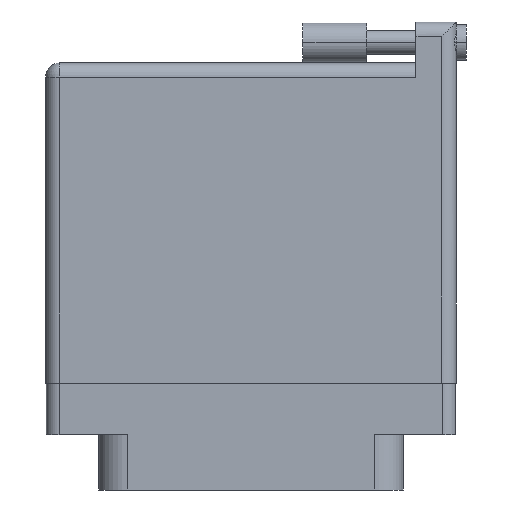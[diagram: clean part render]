
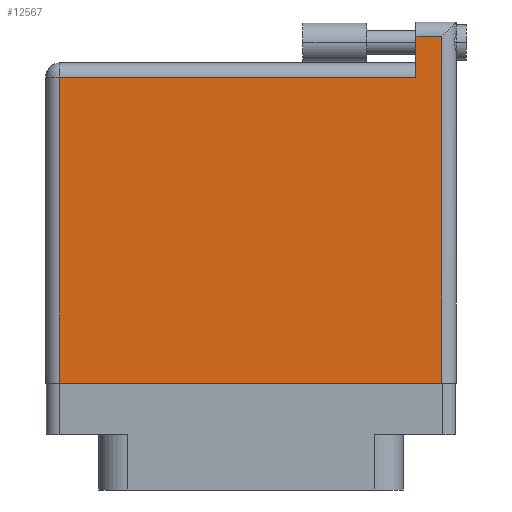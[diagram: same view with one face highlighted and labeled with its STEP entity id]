
A CAD part, front view. The second image highlights one B-rep face of the part: STEP entity #12567.
In plain terms, the highlighted face is planar.
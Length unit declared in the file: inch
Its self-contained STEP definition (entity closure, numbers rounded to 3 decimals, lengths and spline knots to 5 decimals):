
#1122 = AXIS2_PLACEMENT_3D ( 'NONE', #3844, #20524, #31777 ) ;
#2271 = CARTESIAN_POINT ( 'NONE',  ( -1.004, -0.1, 0.4495 ) ) ;
#3331 = CARTESIAN_POINT ( 'NONE',  ( 0.807, 1.396, 0.4495 ) ) ;
#3644 = VERTEX_POINT ( 'NONE', #14735 ) ;
#3844 = CARTESIAN_POINT ( 'NONE',  ( -1.004, 1.466, 0.4495 ) ) ;
#4239 = LINE ( 'NONE', #25022, #27142 ) ;
#4873 = CARTESIAN_POINT ( 'NONE',  ( -0.934, 1.396, 0.4495 ) ) ;
#5853 = EDGE_CURVE ( 'NONE', #35288, #7859, #4239, .T. ) ;
#6407 = LINE ( 'NONE', #24584, #34518 ) ;
#7729 = VECTOR ( 'NONE', #14345, 39.37008 ) ;
#7859 = VERTEX_POINT ( 'NONE', #13746 ) ;
#8720 = CARTESIAN_POINT ( 'NONE',  ( -1.004, 1.596, 0.4495 ) ) ;
#10800 = DIRECTION ( 'NONE',  ( -1., 0., 0. ) ) ;
#11181 = LINE ( 'NONE', #2271, #7729 ) ;
#11555 = EDGE_CURVE ( 'NONE', #15676, #23995, #20229, .T. ) ;
#11770 = DIRECTION ( 'NONE',  ( 0., -1., 0. ) ) ;
#12567 = ADVANCED_FACE ( 'NONE', ( #20068 ), #31891, .F. ) ;
#13208 = EDGE_CURVE ( 'NONE', #7859, #15676, #24707, .T. ) ;
#13276 = ORIENTED_EDGE ( 'NONE', *, *, #21025, .T. ) ;
#13746 = CARTESIAN_POINT ( 'NONE',  ( 0.934, 1.596, 0.4495 ) ) ;
#13770 = CARTESIAN_POINT ( 'NONE',  ( 0.807, 1.596, 0.4495 ) ) ;
#14345 = DIRECTION ( 'NONE',  ( 1., 0., 0. ) ) ;
#14735 = CARTESIAN_POINT ( 'NONE',  ( -0.934, -0.1, 0.4495 ) ) ;
#15373 = VECTOR ( 'NONE', #35369, 39.37008 ) ;
#15676 = VERTEX_POINT ( 'NONE', #13770 ) ;
#17368 = VECTOR ( 'NONE', #28451, 39.37008 ) ;
#19566 = VERTEX_POINT ( 'NONE', #4873 ) ;
#20068 = FACE_OUTER_BOUND ( 'NONE', #30067, .T. ) ;
#20229 = LINE ( 'NONE', #33767, #28402 ) ;
#20524 = DIRECTION ( 'NONE',  ( 0., 0., -1. ) ) ;
#20881 = CARTESIAN_POINT ( 'NONE',  ( 0.934, -0.1, 0.4495 ) ) ;
#21025 = EDGE_CURVE ( 'NONE', #23995, #19566, #6407, .T. ) ;
#23995 = VERTEX_POINT ( 'NONE', #3331 ) ;
#24017 = ORIENTED_EDGE ( 'NONE', *, *, #11555, .T. ) ;
#24584 = CARTESIAN_POINT ( 'NONE',  ( -1.004, 1.396, 0.4495 ) ) ;
#24707 = LINE ( 'NONE', #8720, #17368 ) ;
#25022 = CARTESIAN_POINT ( 'NONE',  ( 0.934, 1.666, 0.4495 ) ) ;
#27142 = VECTOR ( 'NONE', #33024, 39.37008 ) ;
#28402 = VECTOR ( 'NONE', #11770, 39.37008 ) ;
#28451 = DIRECTION ( 'NONE',  ( -1., 0., 0. ) ) ;
#28636 = ORIENTED_EDGE ( 'NONE', *, *, #33900, .T. ) ;
#30067 = EDGE_LOOP ( 'NONE', ( #28636, #32297, #30885, #24017, #13276, #30300 ) ) ;
#30300 = ORIENTED_EDGE ( 'NONE', *, *, #30344, .T. ) ;
#30344 = EDGE_CURVE ( 'NONE', #19566, #3644, #34337, .T. ) ;
#30885 = ORIENTED_EDGE ( 'NONE', *, *, #13208, .T. ) ;
#31777 = DIRECTION ( 'NONE',  ( -1., 0., 0. ) ) ;
#31891 = PLANE ( 'NONE',  #1122 ) ;
#32297 = ORIENTED_EDGE ( 'NONE', *, *, #5853, .T. ) ;
#32622 = CARTESIAN_POINT ( 'NONE',  ( -0.934, -0.1, 0.4495 ) ) ;
#33024 = DIRECTION ( 'NONE',  ( 0., 1., 0. ) ) ;
#33767 = CARTESIAN_POINT ( 'NONE',  ( 0.807, 1.666, 0.4495 ) ) ;
#33900 = EDGE_CURVE ( 'NONE', #3644, #35288, #11181, .T. ) ;
#34337 = LINE ( 'NONE', #32622, #15373 ) ;
#34518 = VECTOR ( 'NONE', #10800, 39.37008 ) ;
#35288 = VERTEX_POINT ( 'NONE', #20881 ) ;
#35369 = DIRECTION ( 'NONE',  ( 0., -1., 0. ) ) ;
